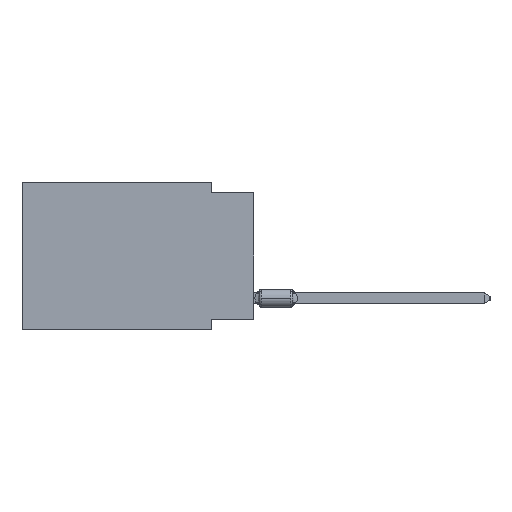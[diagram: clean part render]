
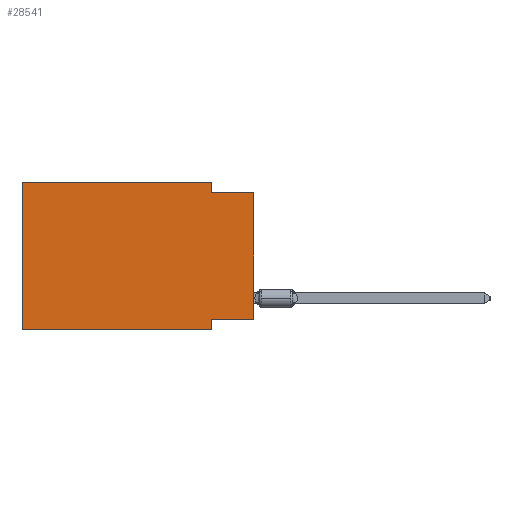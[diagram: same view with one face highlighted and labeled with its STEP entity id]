
A CAD part, left-side view. The second image highlights one B-rep face of the part: STEP entity #28541.
In plain terms, the highlighted planar face has unit normal (-1, 0, 0).
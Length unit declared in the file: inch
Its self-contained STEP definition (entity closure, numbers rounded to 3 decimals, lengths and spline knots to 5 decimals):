
#446 = DIRECTION ( 'NONE',  ( 0., 0., -1. ) ) ;
#666 = CARTESIAN_POINT ( 'NONE',  ( 0., 0.55, 0. ) ) ;
#1926 = CARTESIAN_POINT ( 'NONE',  ( 0., 0., 0. ) ) ;
#1980 = DIRECTION ( 'NONE',  ( 0., -1., 0. ) ) ;
#3002 = CARTESIAN_POINT ( 'NONE',  ( 0., 0.55, 0. ) ) ;
#3377 = VECTOR ( 'NONE', #43628, 39.37008 ) ;
#3692 = VERTEX_POINT ( 'NONE', #34947 ) ;
#3870 = CARTESIAN_POINT ( 'NONE',  ( 0., 0.1, -0.35 ) ) ;
#4968 = LINE ( 'NONE', #15527, #3377 ) ;
#7699 = VECTOR ( 'NONE', #446, 39.37008 ) ;
#8734 = VECTOR ( 'NONE', #25889, 39.37008 ) ;
#8961 = CARTESIAN_POINT ( 'NONE',  ( 0., 0.55, -0.35 ) ) ;
#10225 = ORIENTED_EDGE ( 'NONE', *, *, #26985, .F. ) ;
#10260 = EDGE_CURVE ( 'NONE', #25363, #29450, #11460, .T. ) ;
#10588 = PLANE ( 'NONE',  #26177 ) ;
#11120 = EDGE_CURVE ( 'NONE', #30011, #3692, #30305, .T. ) ;
#11246 = EDGE_CURVE ( 'NONE', #19425, #31954, #27035, .T. ) ;
#11460 = LINE ( 'NONE', #3002, #21101 ) ;
#11502 = LINE ( 'NONE', #3870, #7699 ) ;
#12095 = VECTOR ( 'NONE', #1980, 39.37008 ) ;
#12359 = CARTESIAN_POINT ( 'NONE',  ( 0., 0.55, -0.35 ) ) ;
#12388 = ORIENTED_EDGE ( 'NONE', *, *, #41214, .F. ) ;
#12578 = VERTEX_POINT ( 'NONE', #19259 ) ;
#15436 = CARTESIAN_POINT ( 'NONE',  ( 0., 0.1, 0. ) ) ;
#15527 = CARTESIAN_POINT ( 'NONE',  ( 0., 0.55, 0. ) ) ;
#16271 = LINE ( 'NONE', #43226, #8734 ) ;
#16891 = VECTOR ( 'NONE', #43002, 39.37008 ) ;
#17753 = FACE_OUTER_BOUND ( 'NONE', #41768, .T. ) ;
#19259 = CARTESIAN_POINT ( 'NONE',  ( 0., 0.1, -0.325 ) ) ;
#19425 = VERTEX_POINT ( 'NONE', #38858 ) ;
#20081 = ORIENTED_EDGE ( 'NONE', *, *, #11120, .T. ) ;
#20092 = ORIENTED_EDGE ( 'NONE', *, *, #11246, .F. ) ;
#20276 = DIRECTION ( 'NONE',  ( 0., -1., 0. ) ) ;
#20545 = LINE ( 'NONE', #25922, #37099 ) ;
#20831 = CARTESIAN_POINT ( 'NONE',  ( 0., 0., -0.325 ) ) ;
#20995 = ORIENTED_EDGE ( 'NONE', *, *, #10260, .F. ) ;
#21101 = VECTOR ( 'NONE', #20276, 39.37008 ) ;
#22221 = CARTESIAN_POINT ( 'NONE',  ( 0., 0., -0.025 ) ) ;
#22443 = VERTEX_POINT ( 'NONE', #20831 ) ;
#25283 = ORIENTED_EDGE ( 'NONE', *, *, #26065, .F. ) ;
#25363 = VERTEX_POINT ( 'NONE', #666 ) ;
#25889 = DIRECTION ( 'NONE',  ( 0., 1., 0. ) ) ;
#25922 = CARTESIAN_POINT ( 'NONE',  ( 0., 0.1, 0. ) ) ;
#26065 = EDGE_CURVE ( 'NONE', #12578, #3692, #11502, .T. ) ;
#26177 = AXIS2_PLACEMENT_3D ( 'NONE', #41531, #31224, #30648 ) ;
#26985 = EDGE_CURVE ( 'NONE', #30011, #25363, #4968, .T. ) ;
#27035 = LINE ( 'NONE', #29099, #16891 ) ;
#28337 = ORIENTED_EDGE ( 'NONE', *, *, #43471, .T. ) ;
#28541 = ADVANCED_FACE ( 'NONE', ( #17753 ), #10588, .F. ) ;
#29099 = CARTESIAN_POINT ( 'NONE',  ( 0., 0., -0.025 ) ) ;
#29450 = VERTEX_POINT ( 'NONE', #15436 ) ;
#30011 = VERTEX_POINT ( 'NONE', #8961 ) ;
#30305 = LINE ( 'NONE', #12359, #12095 ) ;
#30648 = DIRECTION ( 'NONE',  ( 0., 0., -1. ) ) ;
#31224 = DIRECTION ( 'NONE',  ( 1., 0., 0. ) ) ;
#31954 = VERTEX_POINT ( 'NONE', #22221 ) ;
#32130 = ORIENTED_EDGE ( 'NONE', *, *, #36343, .F. ) ;
#32569 = VECTOR ( 'NONE', #39034, 39.37008 ) ;
#33678 = LINE ( 'NONE', #1926, #32569 ) ;
#34947 = CARTESIAN_POINT ( 'NONE',  ( 0., 0.1, -0.35 ) ) ;
#36343 = EDGE_CURVE ( 'NONE', #29450, #19425, #20545, .T. ) ;
#37099 = VECTOR ( 'NONE', #39514, 39.37008 ) ;
#38858 = CARTESIAN_POINT ( 'NONE',  ( 0., 0.1, -0.025 ) ) ;
#39034 = DIRECTION ( 'NONE',  ( 0., 0., 1. ) ) ;
#39514 = DIRECTION ( 'NONE',  ( 0., 0., -1. ) ) ;
#41214 = EDGE_CURVE ( 'NONE', #22443, #12578, #16271, .T. ) ;
#41531 = CARTESIAN_POINT ( 'NONE',  ( 0., 0.55, 0. ) ) ;
#41768 = EDGE_LOOP ( 'NONE', ( #28337, #20092, #32130, #20995, #10225, #20081, #25283, #12388 ) ) ;
#43002 = DIRECTION ( 'NONE',  ( 0., -1., 0. ) ) ;
#43226 = CARTESIAN_POINT ( 'NONE',  ( 0., 0., -0.325 ) ) ;
#43471 = EDGE_CURVE ( 'NONE', #22443, #31954, #33678, .T. ) ;
#43628 = DIRECTION ( 'NONE',  ( 0., 0., 1. ) ) ;
